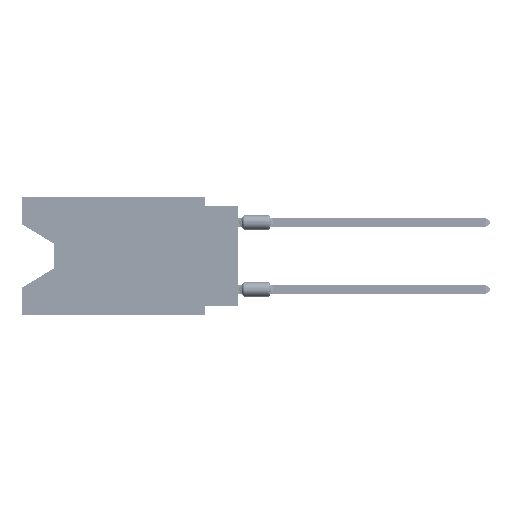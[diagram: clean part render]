
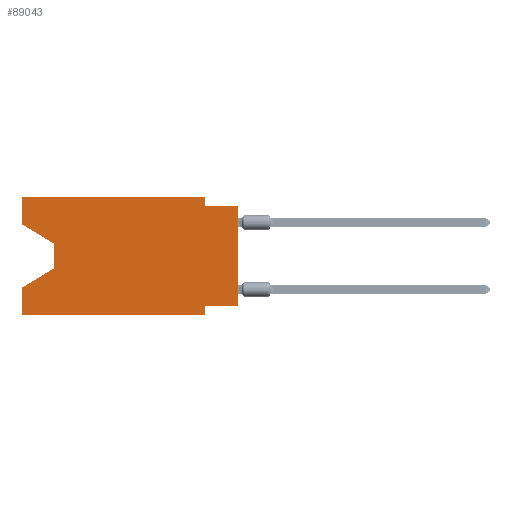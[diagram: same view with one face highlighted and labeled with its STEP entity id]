
A CAD part, left-side view. The second image highlights one B-rep face of the part: STEP entity #89043.
In plain terms, the highlighted planar face has unit normal (-1, 0, 0).
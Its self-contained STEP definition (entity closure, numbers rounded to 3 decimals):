
#3180 = LINE ( 'NONE', #72297, #67583 ) ;
#6156 = CARTESIAN_POINT ( 'NONE',  ( 0., 2.54, -8.255 ) ) ;
#6215 = VERTEX_POINT ( 'NONE', #76392 ) ;
#7667 = CARTESIAN_POINT ( 'NONE',  ( 0., 2.54, -0.635 ) ) ;
#10333 = LINE ( 'NONE', #40008, #57057 ) ;
#10442 = CARTESIAN_POINT ( 'NONE',  ( 0., 0., -0.635 ) ) ;
#11313 = VERTEX_POINT ( 'NONE', #6156 ) ;
#13042 = DIRECTION ( 'NONE',  ( 0., -0.855, -0.519 ) ) ;
#13263 = CARTESIAN_POINT ( 'NONE',  ( 0., 16.383, -2.038 ) ) ;
#13412 = CARTESIAN_POINT ( 'NONE',  ( 0., 16.383, 0. ) ) ;
#13664 = EDGE_CURVE ( 'NONE', #48874, #37074, #10333, .T. ) ;
#14008 = CARTESIAN_POINT ( 'NONE',  ( 0., 0., -0.635 ) ) ;
#14190 = CARTESIAN_POINT ( 'NONE',  ( 0., 16.383, 0. ) ) ;
#15531 = DIRECTION ( 'NONE',  ( 0., 0., 1. ) ) ;
#16227 = DIRECTION ( 'NONE',  ( 0., 0., -1. ) ) ;
#17060 = EDGE_CURVE ( 'NONE', #23522, #23551, #76806, .T. ) ;
#18150 = CARTESIAN_POINT ( 'NONE',  ( 0., 0., 0. ) ) ;
#20370 = DIRECTION ( 'NONE',  ( 0., 0., 1. ) ) ;
#21081 = VECTOR ( 'NONE', #15531, 1000. ) ;
#22232 = ORIENTED_EDGE ( 'NONE', *, *, #44612, .F. ) ;
#22710 = CARTESIAN_POINT ( 'NONE',  ( 0., 2.54, 0. ) ) ;
#23374 = DIRECTION ( 'NONE',  ( 0., 0., -1. ) ) ;
#23522 = VERTEX_POINT ( 'NONE', #13263 ) ;
#23551 = VERTEX_POINT ( 'NONE', #25927 ) ;
#23767 = EDGE_CURVE ( 'NONE', #85839, #64076, #25375, .T. ) ;
#24625 = VECTOR ( 'NONE', #23374, 1000. ) ;
#25375 = LINE ( 'NONE', #18150, #72462 ) ;
#25927 = CARTESIAN_POINT ( 'NONE',  ( 0., 16.383, 0. ) ) ;
#28682 = ORIENTED_EDGE ( 'NONE', *, *, #77359, .F. ) ;
#29353 = CARTESIAN_POINT ( 'NONE',  ( 0., 16.383, 0. ) ) ;
#32823 = VECTOR ( 'NONE', #20370, 1000. ) ;
#33344 = LINE ( 'NONE', #60901, #46408 ) ;
#35686 = DIRECTION ( 'NONE',  ( 1., 0., 0. ) ) ;
#36288 = VECTOR ( 'NONE', #41563, 1000. ) ;
#37074 = VERTEX_POINT ( 'NONE', #7667 ) ;
#38510 = ORIENTED_EDGE ( 'NONE', *, *, #13664, .F. ) ;
#38891 = LINE ( 'NONE', #66442, #77841 ) ;
#39035 = EDGE_CURVE ( 'NONE', #71660, #85538, #3180, .T. ) ;
#39212 = ORIENTED_EDGE ( 'NONE', *, *, #64613, .T. ) ;
#39913 = CARTESIAN_POINT ( 'NONE',  ( 0., 13.97, -3.505 ) ) ;
#40008 = CARTESIAN_POINT ( 'NONE',  ( 0., 2.54, 0. ) ) ;
#40607 = VECTOR ( 'NONE', #87986, 1000. ) ;
#40773 = ORIENTED_EDGE ( 'NONE', *, *, #51831, .F. ) ;
#41003 = CARTESIAN_POINT ( 'NONE',  ( 0., 0., -8.255 ) ) ;
#41411 = DIRECTION ( 'NONE',  ( 0., -1., 0. ) ) ;
#41563 = DIRECTION ( 'NONE',  ( 0., -1., 0. ) ) ;
#41641 = VERTEX_POINT ( 'NONE', #39913 ) ;
#42456 = FACE_OUTER_BOUND ( 'NONE', #63456, .T. ) ;
#43364 = EDGE_CURVE ( 'NONE', #23522, #41641, #47372, .T. ) ;
#44612 = EDGE_CURVE ( 'NONE', #71660, #64785, #48068, .T. ) ;
#44832 = ORIENTED_EDGE ( 'NONE', *, *, #61815, .T. ) ;
#46408 = VECTOR ( 'NONE', #47345, 1000. ) ;
#47345 = DIRECTION ( 'NONE',  ( 0., 1., 0. ) ) ;
#47372 = LINE ( 'NONE', #74935, #68789 ) ;
#47614 = CARTESIAN_POINT ( 'NONE',  ( 0., 16.383, -8.89 ) ) ;
#47747 = LINE ( 'NONE', #13412, #55144 ) ;
#48068 = LINE ( 'NONE', #14190, #21081 ) ;
#48531 = ORIENTED_EDGE ( 'NONE', *, *, #81175, .F. ) ;
#48874 = VERTEX_POINT ( 'NONE', #22710 ) ;
#51831 = EDGE_CURVE ( 'NONE', #23551, #48874, #47747, .T. ) ;
#52823 = ORIENTED_EDGE ( 'NONE', *, *, #17060, .F. ) ;
#53450 = ORIENTED_EDGE ( 'NONE', *, *, #64805, .F. ) ;
#53783 = DIRECTION ( 'NONE',  ( 0., 0., -1. ) ) ;
#55144 = VECTOR ( 'NONE', #41411, 1000. ) ;
#57057 = VECTOR ( 'NONE', #85762, 1000. ) ;
#57422 = DIRECTION ( 'NONE',  ( 0., -1., 0. ) ) ;
#60901 = CARTESIAN_POINT ( 'NONE',  ( 0., 0., -8.255 ) ) ;
#61815 = EDGE_CURVE ( 'NONE', #41641, #6215, #85677, .T. ) ;
#63104 = ORIENTED_EDGE ( 'NONE', *, *, #43364, .T. ) ;
#63456 = EDGE_LOOP ( 'NONE', ( #63104, #44832, #39212, #22232, #67083, #28682, #53450, #65091, #48531, #38510, #40773, #52823 ) ) ;
#64076 = VERTEX_POINT ( 'NONE', #10442 ) ;
#64613 = EDGE_CURVE ( 'NONE', #6215, #64785, #73556, .T. ) ;
#64785 = VERTEX_POINT ( 'NONE', #75346 ) ;
#64805 = EDGE_CURVE ( 'NONE', #85839, #11313, #33344, .T. ) ;
#65091 = ORIENTED_EDGE ( 'NONE', *, *, #23767, .T. ) ;
#65427 = CARTESIAN_POINT ( 'NONE',  ( 0., 13.97, -5.385 ) ) ;
#66442 = CARTESIAN_POINT ( 'NONE',  ( 0., 2.54, -8.89 ) ) ;
#67083 = ORIENTED_EDGE ( 'NONE', *, *, #39035, .T. ) ;
#67583 = VECTOR ( 'NONE', #57422, 1000. ) ;
#68789 = VECTOR ( 'NONE', #13042, 1000. ) ;
#69124 = LINE ( 'NONE', #14008, #36288 ) ;
#70905 = CARTESIAN_POINT ( 'NONE',  ( 0., 2.54, -8.89 ) ) ;
#71660 = VERTEX_POINT ( 'NONE', #47614 ) ;
#72297 = CARTESIAN_POINT ( 'NONE',  ( 0., 16.383, -8.89 ) ) ;
#72366 = DIRECTION ( 'NONE',  ( 0., 0., 1. ) ) ;
#72462 = VECTOR ( 'NONE', #72366, 1000. ) ;
#73556 = LINE ( 'NONE', #65427, #40607 ) ;
#74935 = CARTESIAN_POINT ( 'NONE',  ( 0., 16.383, -2.038 ) ) ;
#75346 = CARTESIAN_POINT ( 'NONE',  ( 0., 16.383, -6.852 ) ) ;
#76392 = CARTESIAN_POINT ( 'NONE',  ( 0., 13.97, -5.385 ) ) ;
#76806 = LINE ( 'NONE', #83127, #32823 ) ;
#77359 = EDGE_CURVE ( 'NONE', #11313, #85538, #38891, .T. ) ;
#77841 = VECTOR ( 'NONE', #53783, 1000. ) ;
#78116 = PLANE ( 'NONE',  #87733 ) ;
#81175 = EDGE_CURVE ( 'NONE', #37074, #64076, #69124, .T. ) ;
#83127 = CARTESIAN_POINT ( 'NONE',  ( 0., 16.383, 0. ) ) ;
#85243 = CARTESIAN_POINT ( 'NONE',  ( 0., 13.97, -3.505 ) ) ;
#85538 = VERTEX_POINT ( 'NONE', #70905 ) ;
#85677 = LINE ( 'NONE', #85243, #24625 ) ;
#85762 = DIRECTION ( 'NONE',  ( 0., 0., -1. ) ) ;
#85839 = VERTEX_POINT ( 'NONE', #41003 ) ;
#87733 = AXIS2_PLACEMENT_3D ( 'NONE', #29353, #35686, #16227 ) ;
#87986 = DIRECTION ( 'NONE',  ( 0., 0.855, -0.519 ) ) ;
#89043 = ADVANCED_FACE ( 'NONE', ( #42456 ), #78116, .F. ) ;
